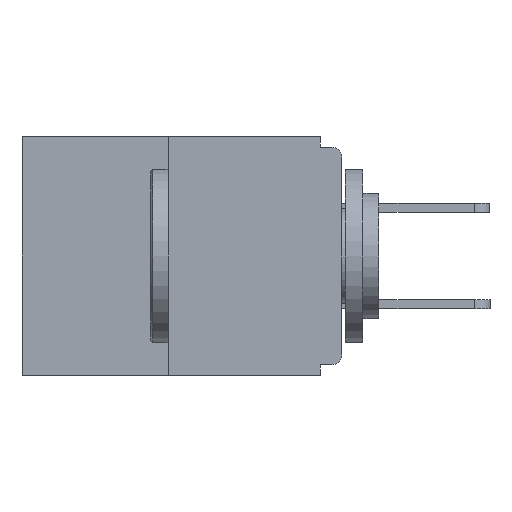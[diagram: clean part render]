
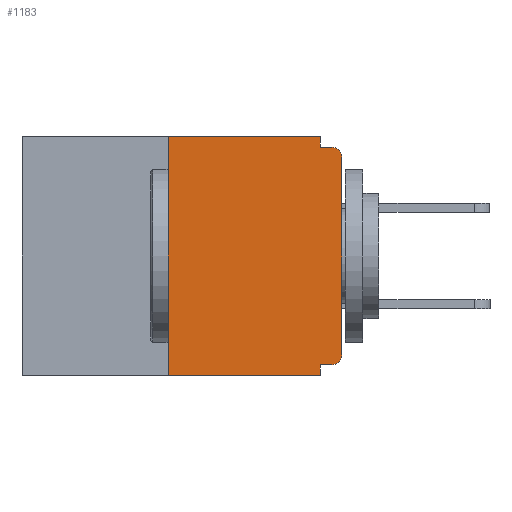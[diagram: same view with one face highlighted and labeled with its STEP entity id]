
A CAD part, left-side view. The second image highlights one B-rep face of the part: STEP entity #1183.
In plain terms, the highlighted planar face has unit normal (-1, 0, 0).
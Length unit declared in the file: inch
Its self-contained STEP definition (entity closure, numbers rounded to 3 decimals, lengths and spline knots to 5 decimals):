
#753 = CARTESIAN_POINT ( 'NONE',  ( 0., 0.25, -0.343 ) ) ;
#928 = FACE_OUTER_BOUND ( 'NONE', #5453, .T. ) ;
#994 = ORIENTED_EDGE ( 'NONE', *, *, #19117, .T. ) ;
#1183 = ADVANCED_FACE ( 'NONE', ( #928 ), #11181, .F. ) ;
#1802 = VERTEX_POINT ( 'NONE', #753 ) ;
#2245 = VERTEX_POINT ( 'NONE', #8095 ) ;
#2827 = DIRECTION ( 'NONE',  ( 0., 1., 0. ) ) ;
#4047 = VERTEX_POINT ( 'NONE', #7526 ) ;
#4170 = VECTOR ( 'NONE', #27740, 39.37008 ) ;
#4442 = VERTEX_POINT ( 'NONE', #20541 ) ;
#4474 = VECTOR ( 'NONE', #5301, 39.37008 ) ;
#4748 = DIRECTION ( 'NONE',  ( 0., 0., -1. ) ) ;
#5234 = LINE ( 'NONE', #22475, #14862 ) ;
#5301 = DIRECTION ( 'NONE',  ( 0., 0., -1. ) ) ;
#5453 = EDGE_LOOP ( 'NONE', ( #27152, #21014, #17835, #24488, #7799, #21238, #994, #14025, #13481, #9127 ) ) ;
#5648 = CARTESIAN_POINT ( 'NONE',  ( 0., 0., -0.03 ) ) ;
#6041 = CARTESIAN_POINT ( 'NONE',  ( 0., 0.015, -0.313 ) ) ;
#6258 = CARTESIAN_POINT ( 'NONE',  ( 0., 0., 0. ) ) ;
#6437 = DIRECTION ( 'NONE',  ( 0., -1., 0. ) ) ;
#6578 = VECTOR ( 'NONE', #6437, 39.37008 ) ;
#6683 = EDGE_CURVE ( 'NONE', #1802, #2245, #18639, .T. ) ;
#7300 = AXIS2_PLACEMENT_3D ( 'NONE', #6041, #11233, #22869 ) ;
#7503 = VECTOR ( 'NONE', #4748, 39.37008 ) ;
#7526 = CARTESIAN_POINT ( 'NONE',  ( 0., 0.015, -0.015 ) ) ;
#7799 = ORIENTED_EDGE ( 'NONE', *, *, #17943, .F. ) ;
#8095 = CARTESIAN_POINT ( 'NONE',  ( 0., 0.25, 0. ) ) ;
#8233 = VERTEX_POINT ( 'NONE', #5648 ) ;
#9127 = ORIENTED_EDGE ( 'NONE', *, *, #25971, .F. ) ;
#9654 = VERTEX_POINT ( 'NONE', #11376 ) ;
#9866 = VERTEX_POINT ( 'NONE', #27325 ) ;
#9987 = LINE ( 'NONE', #25315, #4474 ) ;
#11104 = CARTESIAN_POINT ( 'NONE',  ( 0., 0.031, -0.343 ) ) ;
#11181 = PLANE ( 'NONE',  #19466 ) ;
#11233 = DIRECTION ( 'NONE',  ( -1., 0., 0. ) ) ;
#11302 = EDGE_CURVE ( 'NONE', #1802, #20617, #16121, .T. ) ;
#11376 = CARTESIAN_POINT ( 'NONE',  ( 0., 0.015, -0.328 ) ) ;
#12422 = LINE ( 'NONE', #6258, #23969 ) ;
#12578 = CARTESIAN_POINT ( 'NONE',  ( 0., 0.46, -0.343 ) ) ;
#12930 = VECTOR ( 'NONE', #19821, 39.37008 ) ;
#13113 = CARTESIAN_POINT ( 'NONE',  ( 0., 0.46, 0. ) ) ;
#13397 = DIRECTION ( 'NONE',  ( 1., 0., 0. ) ) ;
#13467 = DIRECTION ( 'NONE',  ( 0., 0., 1. ) ) ;
#13481 = ORIENTED_EDGE ( 'NONE', *, *, #18747, .F. ) ;
#13603 = CIRCLE ( 'NONE', #20956, 0.015 ) ;
#13687 = CARTESIAN_POINT ( 'NONE',  ( 0., 0., -0.313 ) ) ;
#13722 = VERTEX_POINT ( 'NONE', #26024 ) ;
#13996 = EDGE_CURVE ( 'NONE', #8233, #4047, #13603, .T. ) ;
#14025 = ORIENTED_EDGE ( 'NONE', *, *, #13996, .T. ) ;
#14818 = DIRECTION ( 'NONE',  ( 0., 0., -1. ) ) ;
#14862 = VECTOR ( 'NONE', #2827, 39.37008 ) ;
#16121 = LINE ( 'NONE', #12578, #4170 ) ;
#17835 = ORIENTED_EDGE ( 'NONE', *, *, #11302, .T. ) ;
#17943 = EDGE_CURVE ( 'NONE', #9654, #13722, #5234, .T. ) ;
#18639 = LINE ( 'NONE', #24143, #12930 ) ;
#18699 = CIRCLE ( 'NONE', #7300, 0.015 ) ;
#18747 = EDGE_CURVE ( 'NONE', #9866, #4047, #19887, .T. ) ;
#18880 = CARTESIAN_POINT ( 'NONE',  ( 0., 0., -0.015 ) ) ;
#18988 = DIRECTION ( 'NONE',  ( 0., -1., 0. ) ) ;
#19117 = EDGE_CURVE ( 'NONE', #25803, #8233, #12422, .T. ) ;
#19466 = AXIS2_PLACEMENT_3D ( 'NONE', #13113, #13397, #24122 ) ;
#19748 = EDGE_CURVE ( 'NONE', #13722, #20617, #24896, .T. ) ;
#19821 = DIRECTION ( 'NONE',  ( 0., 0., 1. ) ) ;
#19887 = LINE ( 'NONE', #18880, #23317 ) ;
#20541 = CARTESIAN_POINT ( 'NONE',  ( 0., 0.031, 0. ) ) ;
#20617 = VERTEX_POINT ( 'NONE', #21362 ) ;
#20947 = CARTESIAN_POINT ( 'NONE',  ( 0., 0.015, -0.03 ) ) ;
#20956 = AXIS2_PLACEMENT_3D ( 'NONE', #20947, #25536, #14818 ) ;
#21014 = ORIENTED_EDGE ( 'NONE', *, *, #6683, .F. ) ;
#21238 = ORIENTED_EDGE ( 'NONE', *, *, #27605, .T. ) ;
#21362 = CARTESIAN_POINT ( 'NONE',  ( 0., 0.031, -0.343 ) ) ;
#22475 = CARTESIAN_POINT ( 'NONE',  ( 0., 0., -0.328 ) ) ;
#22869 = DIRECTION ( 'NONE',  ( 0., 0., -1. ) ) ;
#23317 = VECTOR ( 'NONE', #18988, 39.37008 ) ;
#23969 = VECTOR ( 'NONE', #13467, 39.37008 ) ;
#24122 = DIRECTION ( 'NONE',  ( 0., 0., -1. ) ) ;
#24143 = CARTESIAN_POINT ( 'NONE',  ( 0., 0.25, 0. ) ) ;
#24488 = ORIENTED_EDGE ( 'NONE', *, *, #19748, .F. ) ;
#24896 = LINE ( 'NONE', #11104, #7503 ) ;
#24910 = EDGE_CURVE ( 'NONE', #2245, #4442, #27386, .T. ) ;
#25315 = CARTESIAN_POINT ( 'NONE',  ( 0., 0.031, 0. ) ) ;
#25536 = DIRECTION ( 'NONE',  ( -1., 0., 0. ) ) ;
#25803 = VERTEX_POINT ( 'NONE', #13687 ) ;
#25971 = EDGE_CURVE ( 'NONE', #4442, #9866, #9987, .T. ) ;
#26024 = CARTESIAN_POINT ( 'NONE',  ( 0., 0.031, -0.328 ) ) ;
#27152 = ORIENTED_EDGE ( 'NONE', *, *, #24910, .F. ) ;
#27325 = CARTESIAN_POINT ( 'NONE',  ( 0., 0.031, -0.015 ) ) ;
#27386 = LINE ( 'NONE', #27994, #6578 ) ;
#27605 = EDGE_CURVE ( 'NONE', #9654, #25803, #18699, .T. ) ;
#27740 = DIRECTION ( 'NONE',  ( 0., -1., 0. ) ) ;
#27994 = CARTESIAN_POINT ( 'NONE',  ( 0., 0.46, 0. ) ) ;
